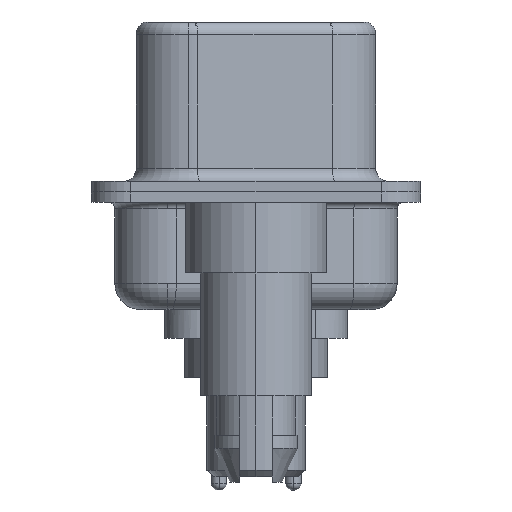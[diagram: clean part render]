
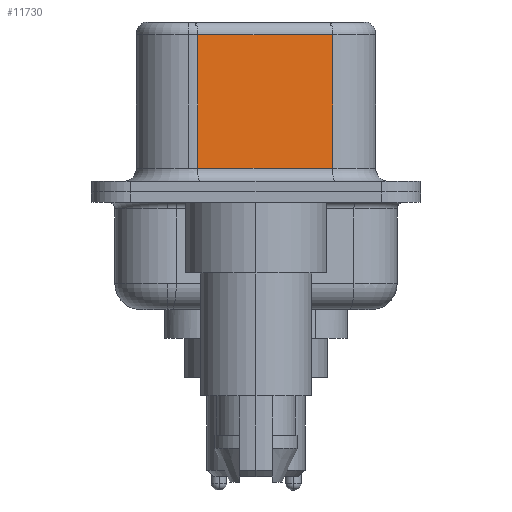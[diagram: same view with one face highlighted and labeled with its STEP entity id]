
A CAD part, left-side view. The second image highlights one B-rep face of the part: STEP entity #11730.
In plain terms, the highlighted planar face has unit normal (-0.985, -0.174, 0).
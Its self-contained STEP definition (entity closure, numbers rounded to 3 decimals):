
#165 = ORIENTED_EDGE ( 'NONE', *, *, #14167, .F. ) ;
#1889 = VECTOR ( 'NONE', #3357, 1000. ) ;
#3357 = DIRECTION ( 'NONE',  ( 0., 0., -1. ) ) ;
#3910 = EDGE_CURVE ( 'NONE', #19034, #15993, #6633, .T. ) ;
#4108 = CARTESIAN_POINT ( 'NONE',  ( 3.67, 2.233, 0.9 ) ) ;
#5841 = VERTEX_POINT ( 'NONE', #4108 ) ;
#6062 = VECTOR ( 'NONE', #11279, 1000. ) ;
#6148 = VECTOR ( 'NONE', #20770, 1000. ) ;
#6633 = LINE ( 'NONE', #22958, #6062 ) ;
#7744 = CARTESIAN_POINT ( 'NONE',  ( 3.67, 2.233, 6.52 ) ) ;
#8410 = PLANE ( 'NONE',  #14487 ) ;
#9316 = CARTESIAN_POINT ( 'NONE',  ( 3.67, 2.233, 6.02 ) ) ;
#9543 = CARTESIAN_POINT ( 'NONE',  ( 4.58, -2.927, 0.9 ) ) ;
#10329 = DIRECTION ( 'NONE',  ( 0.985, 0.174, 0. ) ) ;
#10512 = CARTESIAN_POINT ( 'NONE',  ( 4.58, -2.927, 6.02 ) ) ;
#11279 = DIRECTION ( 'NONE',  ( -0.174, 0.985, 0. ) ) ;
#11730 = ADVANCED_FACE ( 'NONE', ( #17530 ), #8410, .F. ) ;
#12153 = EDGE_LOOP ( 'NONE', ( #165, #20099, #22254, #19952 ) ) ;
#14167 = EDGE_CURVE ( 'NONE', #19034, #20179, #16251, .T. ) ;
#14241 = EDGE_CURVE ( 'NONE', #5841, #20179, #15089, .T. ) ;
#14487 = AXIS2_PLACEMENT_3D ( 'NONE', #21405, #10329, #23239 ) ;
#15089 = LINE ( 'NONE', #9543, #19982 ) ;
#15993 = VERTEX_POINT ( 'NONE', #9316 ) ;
#16094 = LINE ( 'NONE', #7744, #6148 ) ;
#16251 = LINE ( 'NONE', #21926, #1889 ) ;
#17530 = FACE_OUTER_BOUND ( 'NONE', #12153, .T. ) ;
#19034 = VERTEX_POINT ( 'NONE', #10512 ) ;
#19327 = EDGE_CURVE ( 'NONE', #15993, #5841, #16094, .T. ) ;
#19952 = ORIENTED_EDGE ( 'NONE', *, *, #14241, .T. ) ;
#19982 = VECTOR ( 'NONE', #22472, 1000. ) ;
#20099 = ORIENTED_EDGE ( 'NONE', *, *, #3910, .T. ) ;
#20179 = VERTEX_POINT ( 'NONE', #20745 ) ;
#20745 = CARTESIAN_POINT ( 'NONE',  ( 4.58, -2.927, 0.9 ) ) ;
#20770 = DIRECTION ( 'NONE',  ( 0., 0., -1. ) ) ;
#21405 = CARTESIAN_POINT ( 'NONE',  ( 4.58, -2.927, 6.52 ) ) ;
#21926 = CARTESIAN_POINT ( 'NONE',  ( 4.58, -2.927, 6.52 ) ) ;
#22254 = ORIENTED_EDGE ( 'NONE', *, *, #19327, .T. ) ;
#22472 = DIRECTION ( 'NONE',  ( 0.174, -0.985, 0. ) ) ;
#22958 = CARTESIAN_POINT ( 'NONE',  ( 4.58, -2.927, 6.02 ) ) ;
#23239 = DIRECTION ( 'NONE',  ( -0.174, 0.985, 0. ) ) ;
